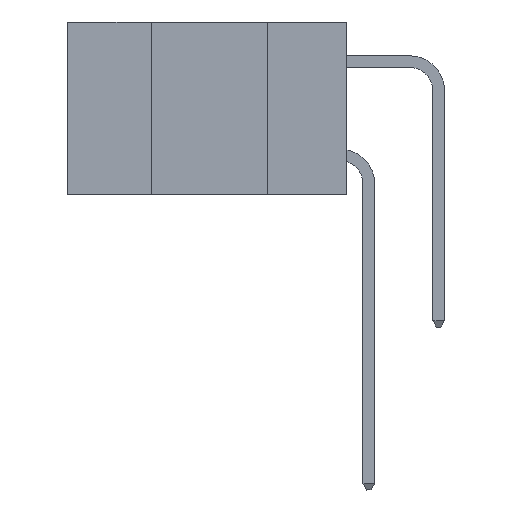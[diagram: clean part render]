
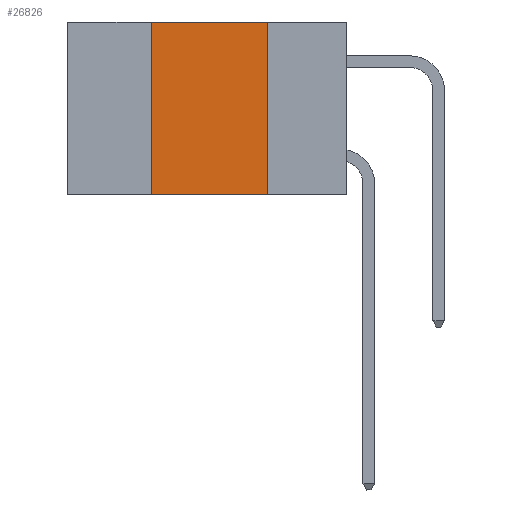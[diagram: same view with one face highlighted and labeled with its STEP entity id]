
A CAD part, left-side view. The second image highlights one B-rep face of the part: STEP entity #26826.
In plain terms, the highlighted planar face has unit normal (-1, 0, 0).
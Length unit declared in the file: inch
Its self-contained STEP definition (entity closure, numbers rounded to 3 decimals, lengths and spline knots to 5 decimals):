
#152 = EDGE_CURVE ( 'NONE', #10405, #17700, #5368, .T. ) ;
#293 = EDGE_CURVE ( 'NONE', #10405, #7356, #11579, .T. ) ;
#974 = CARTESIAN_POINT ( 'NONE',  ( 0., 0.6, 0. ) ) ;
#1058 = CARTESIAN_POINT ( 'NONE',  ( 0., 0.17, 0. ) ) ;
#1719 = CARTESIAN_POINT ( 'NONE',  ( 0., 0.6, -0.37 ) ) ;
#2409 = CARTESIAN_POINT ( 'NONE',  ( 0., 0.17, 0. ) ) ;
#2558 = EDGE_CURVE ( 'NONE', #17700, #4268, #20464, .T. ) ;
#3105 = VECTOR ( 'NONE', #8139, 39.37008 ) ;
#4102 = DIRECTION ( 'NONE',  ( 0., -1., 0. ) ) ;
#4268 = VERTEX_POINT ( 'NONE', #1058 ) ;
#5368 = LINE ( 'NONE', #7637, #18680 ) ;
#7356 = VERTEX_POINT ( 'NONE', #17637 ) ;
#7637 = CARTESIAN_POINT ( 'NONE',  ( 0., 0.42, 0. ) ) ;
#8139 = DIRECTION ( 'NONE',  ( 0., -1., 0. ) ) ;
#8369 = ORIENTED_EDGE ( 'NONE', *, *, #293, .T. ) ;
#9169 = CARTESIAN_POINT ( 'NONE',  ( 0., 0.42, 0. ) ) ;
#9437 = VECTOR ( 'NONE', #4102, 39.37008 ) ;
#10405 = VERTEX_POINT ( 'NONE', #20756 ) ;
#10729 = EDGE_LOOP ( 'NONE', ( #18262, #25090, #25087, #8369 ) ) ;
#11579 = LINE ( 'NONE', #1719, #3105 ) ;
#12023 = DIRECTION ( 'NONE',  ( 0., 0., 1. ) ) ;
#12384 = CARTESIAN_POINT ( 'NONE',  ( 0., 0.6, 0. ) ) ;
#16399 = EDGE_CURVE ( 'NONE', #4268, #7356, #18844, .T. ) ;
#17547 = DIRECTION ( 'NONE',  ( 0., 0., -1. ) ) ;
#17637 = CARTESIAN_POINT ( 'NONE',  ( 0., 0.17, -0.37 ) ) ;
#17700 = VERTEX_POINT ( 'NONE', #9169 ) ;
#18262 = ORIENTED_EDGE ( 'NONE', *, *, #16399, .F. ) ;
#18680 = VECTOR ( 'NONE', #12023, 39.37008 ) ;
#18720 = DIRECTION ( 'NONE',  ( 0., 0., -1. ) ) ;
#18844 = LINE ( 'NONE', #2409, #20144 ) ;
#20144 = VECTOR ( 'NONE', #18720, 39.37008 ) ;
#20464 = LINE ( 'NONE', #12384, #9437 ) ;
#20756 = CARTESIAN_POINT ( 'NONE',  ( 0., 0.42, -0.37 ) ) ;
#20995 = PLANE ( 'NONE',  #21685 ) ;
#21685 = AXIS2_PLACEMENT_3D ( 'NONE', #974, #23557, #17547 ) ;
#23557 = DIRECTION ( 'NONE',  ( 1., 0., 0. ) ) ;
#25087 = ORIENTED_EDGE ( 'NONE', *, *, #152, .F. ) ;
#25090 = ORIENTED_EDGE ( 'NONE', *, *, #2558, .F. ) ;
#26584 = FACE_OUTER_BOUND ( 'NONE', #10729, .T. ) ;
#26826 = ADVANCED_FACE ( 'NONE', ( #26584 ), #20995, .F. ) ;
